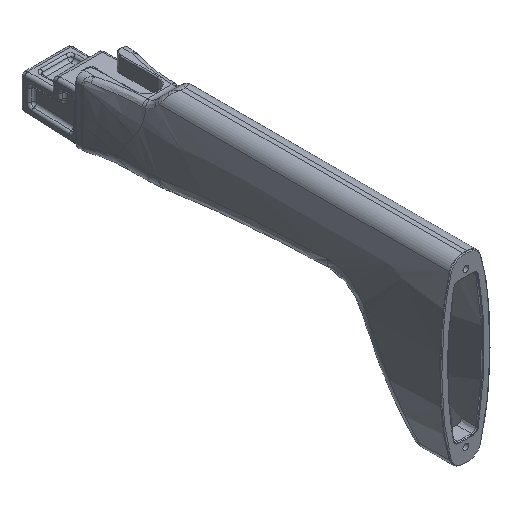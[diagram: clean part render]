
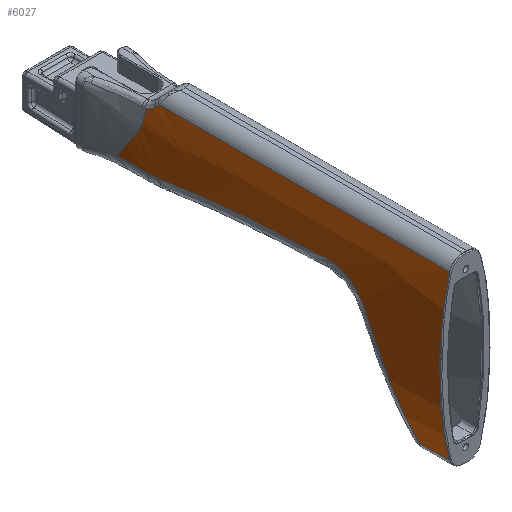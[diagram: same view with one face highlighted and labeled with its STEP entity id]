
A CAD part, isometric view. The second image highlights one B-rep face of the part: STEP entity #6027.
In plain terms, the highlighted free-form (B-spline) face has degree [1, 2] with [2, 5] control points.
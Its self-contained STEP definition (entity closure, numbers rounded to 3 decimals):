
#101=B_SPLINE_CURVE_WITH_KNOTS('',3,(#11541,#11542,#11543,#11544),
 .UNSPECIFIED.,.F.,.F.,(4,4),(-0.253,0.),.UNSPECIFIED.);
#102=B_SPLINE_CURVE_WITH_KNOTS('',3,(#11589,#11590,#11591,#11592,#11593,
#11594,#11595),.UNSPECIFIED.,.F.,.F.,(4,1,1,1,4),(-6.528,-5.596,
-4.663,-2.798,0.),.UNSPECIFIED.);
#103=B_SPLINE_CURVE_WITH_KNOTS('',3,(#11634,#11635,#11636,#11637,#11638,
#11639),.UNSPECIFIED.,.F.,.F.,(4,1,1,4),(-3.312,-2.366,
-1.419,0.),.UNSPECIFIED.);
#104=B_SPLINE_CURVE_WITH_KNOTS('',3,(#11666,#11667,#11668,#11669),
 .UNSPECIFIED.,.F.,.F.,(4,4),(-10.9,0.),.UNSPECIFIED.);
#105=B_SPLINE_CURVE_WITH_KNOTS('',3,(#11696,#11697,#11698,#11699),
 .UNSPECIFIED.,.F.,.F.,(4,4),(-0.712,0.),.UNSPECIFIED.);
#106=B_SPLINE_CURVE_WITH_KNOTS('',3,(#11724,#11725,#11726,#11727,#11728),
 .UNSPECIFIED.,.F.,.F.,(4,1,4),(23.985,24.996,26.344),
 .UNSPECIFIED.);
#107=B_SPLINE_CURVE_WITH_KNOTS('',3,(#11758,#11759,#11760,#11761,#11762,
#11763),.UNSPECIFIED.,.F.,.F.,(4,1,1,4),(0.,0.978,2.933,
3.125),.UNSPECIFIED.);
#108=B_SPLINE_CURVE_WITH_KNOTS('',3,(#11785,#11786,#11787,#11788),
 .UNSPECIFIED.,.F.,.F.,(4,4),(-0.662,-0.338),
 .UNSPECIFIED.);
#109=B_SPLINE_CURVE_WITH_KNOTS('',3,(#11789,#11790,#11791,#11792),
 .UNSPECIFIED.,.F.,.F.,(4,4),(-0.338,0.),.UNSPECIFIED.);
#124=B_SPLINE_CURVE_WITH_KNOTS('',3,(#12249,#12250,#12251,#12252,#12253,
#12254,#12255,#12256,#12257,#12258,#12259),.UNSPECIFIED.,.F.,.F.,(4,1,1,
1,1,1,1,1,4),(0.,0.763,1.525,3.05,4.575,
7.626,9.151,9.913,10.676),
 .UNSPECIFIED.);
#488=(
BOUNDED_SURFACE()
B_SPLINE_SURFACE(1,2,((#12238,#12239,#12240,#12241,#12242),(#12243,#12244,
#12245,#12246,#12247)),.UNSPECIFIED.,.F.,.F.,.F.)
B_SPLINE_SURFACE_WITH_KNOTS((2,2),(3,2,3),(0.041,3.152),
(-2.476,-1.571,-0.665),.UNSPECIFIED.)
GEOMETRIC_REPRESENTATION_ITEM()
RATIONAL_B_SPLINE_SURFACE(((1.,0.899,1.,0.899,1.),
(1.,0.899,1.,0.899,1.)))
REPRESENTATION_ITEM('')
SURFACE()
);
#880=FACE_OUTER_BOUND('',#1303,.T.);
#1303=EDGE_LOOP('',(#4921,#4922,#4923,#4924,#4925,#4926,#4927,#4928,#4929,
#4930,#4931,#4932,#4933));
#1636=LINE('',#11702,#1891);
#1640=LINE('',#12236,#1895);
#1642=LINE('',#12260,#1897);
#1891=VECTOR('',#7911,10.);
#1895=VECTOR('',#7957,10.);
#1897=VECTOR('',#7959,10.);
#2610=VERTEX_POINT('',#10348);
#2615=VERTEX_POINT('',#10564);
#2659=VERTEX_POINT('',#11513);
#2661=VERTEX_POINT('',#11538);
#2662=VERTEX_POINT('',#11540);
#2663=VERTEX_POINT('',#11588);
#2664=VERTEX_POINT('',#11633);
#2665=VERTEX_POINT('',#11665);
#2666=VERTEX_POINT('',#11695);
#2667=VERTEX_POINT('',#11723);
#2668=VERTEX_POINT('',#11784);
#2684=VERTEX_POINT('',#12233);
#2686=VERTEX_POINT('',#12248);
#3407=EDGE_CURVE('',#2661,#2662,#101,.T.);
#3409=EDGE_CURVE('',#2659,#2663,#102,.T.);
#3411=EDGE_CURVE('',#2663,#2664,#103,.T.);
#3413=EDGE_CURVE('',#2664,#2665,#104,.T.);
#3415=EDGE_CURVE('',#2665,#2666,#105,.T.);
#3417=EDGE_CURVE('',#2666,#2610,#1636,.T.);
#3418=EDGE_CURVE('',#2610,#2667,#106,.T.);
#3420=EDGE_CURVE('',#2667,#2615,#107,.T.);
#3421=EDGE_CURVE('',#2615,#2668,#108,.T.);
#3422=EDGE_CURVE('',#2668,#2661,#109,.T.);
#3455=EDGE_CURVE('',#2659,#2684,#1640,.T.);
#3457=EDGE_CURVE('',#2686,#2684,#124,.T.);
#3458=EDGE_CURVE('',#2686,#2662,#1642,.T.);
#4921=ORIENTED_EDGE('',*,*,#3421,.F.);
#4922=ORIENTED_EDGE('',*,*,#3420,.F.);
#4923=ORIENTED_EDGE('',*,*,#3418,.F.);
#4924=ORIENTED_EDGE('',*,*,#3417,.F.);
#4925=ORIENTED_EDGE('',*,*,#3415,.F.);
#4926=ORIENTED_EDGE('',*,*,#3413,.F.);
#4927=ORIENTED_EDGE('',*,*,#3411,.F.);
#4928=ORIENTED_EDGE('',*,*,#3409,.F.);
#4929=ORIENTED_EDGE('',*,*,#3455,.T.);
#4930=ORIENTED_EDGE('',*,*,#3457,.F.);
#4931=ORIENTED_EDGE('',*,*,#3458,.T.);
#4932=ORIENTED_EDGE('',*,*,#3407,.F.);
#4933=ORIENTED_EDGE('',*,*,#3422,.F.);
#6027=ADVANCED_FACE('',(#880),#488,.T.);
#7911=DIRECTION('',(0.,1.,0.));
#7957=DIRECTION('',(0.,-1.,0.));
#7959=DIRECTION('',(0.,1.,0.));
#10348=CARTESIAN_POINT('',(-15.76,-485.341,96.708));
#10564=CARTESIAN_POINT('',(-11.416,-499.135,128.202));
#11513=CARTESIAN_POINT('',(-10.031,-674.92,27.353));
#11538=CARTESIAN_POINT('',(-10.569,-504.818,131.424));
#11540=CARTESIAN_POINT('',(-10.031,-506.567,133.253));
#11541=CARTESIAN_POINT('Ctrl Pts',(-10.569,-504.818,
131.424));
#11542=CARTESIAN_POINT('Ctrl Pts',(-10.398,-505.402,132.033));
#11543=CARTESIAN_POINT('Ctrl Pts',(-10.219,-505.985,
132.643));
#11544=CARTESIAN_POINT('Ctrl Pts',(-10.031,-506.567,133.253));
#11588=CARTESIAN_POINT('',(-16.12,-647.054,88.811));
#11589=CARTESIAN_POINT('Ctrl Pts',(-10.031,-674.92,27.353));
#11590=CARTESIAN_POINT('Ctrl Pts',(-10.976,-673.632,
30.426));
#11591=CARTESIAN_POINT('Ctrl Pts',(-12.421,-671.02,
36.399));
#11592=CARTESIAN_POINT('Ctrl Pts',(-14.446,-665.738,
48.158));
#11593=CARTESIAN_POINT('Ctrl Pts',(-16.163,-657.746,
65.617));
#11594=CARTESIAN_POINT('Ctrl Pts',(-16.387,-651.061,80.106));
#11595=CARTESIAN_POINT('Ctrl Pts',(-16.12,-647.054,
88.811));
#11633=CARTESIAN_POINT('',(-15.023,-620.438,105.958));
#11634=CARTESIAN_POINT('Ctrl Pts',(-16.12,-647.054,
88.811));
#11635=CARTESIAN_POINT('Ctrl Pts',(-16.029,-645.699,
91.755));
#11636=CARTESIAN_POINT('Ctrl Pts',(-15.766,-642.052,97.18));
#11637=CARTESIAN_POINT('Ctrl Pts',(-15.225,-633.073,
104.094));
#11638=CARTESIAN_POINT('Ctrl Pts',(-15.016,-625.169,106.031));
#11639=CARTESIAN_POINT('Ctrl Pts',(-15.023,-620.438,
105.958));
#11665=CARTESIAN_POINT('',(-15.728,-511.831,97.222));
#11666=CARTESIAN_POINT('Ctrl Pts',(-15.023,-620.438,
105.958));
#11667=CARTESIAN_POINT('Ctrl Pts',(-15.079,-584.107,
105.394));
#11668=CARTESIAN_POINT('Ctrl Pts',(-15.399,-547.811,102.464));
#11669=CARTESIAN_POINT('Ctrl Pts',(-15.728,-511.831,
97.222));
#11695=CARTESIAN_POINT('',(-15.76,-504.734,96.708));
#11696=CARTESIAN_POINT('Ctrl Pts',(-15.728,-511.831,
97.222));
#11697=CARTESIAN_POINT('Ctrl Pts',(-15.75,-509.481,
96.88));
#11698=CARTESIAN_POINT('Ctrl Pts',(-15.76,-507.108,
96.708));
#11699=CARTESIAN_POINT('Ctrl Pts',(-15.76,-504.734,
96.708));
#11702=CARTESIAN_POINT('',(-15.76,-697.501,96.708));
#11723=CARTESIAN_POINT('',(-14.433,-494.201,111.229));
#11724=CARTESIAN_POINT('Ctrl Pts',(-15.76,-485.341,
96.708));
#11725=CARTESIAN_POINT('Ctrl Pts',(-15.626,-486.392,
98.922));
#11726=CARTESIAN_POINT('Ctrl Pts',(-15.251,-489.155,
103.977));
#11727=CARTESIAN_POINT('Ctrl Pts',(-14.754,-492.311,
108.661));
#11728=CARTESIAN_POINT('Ctrl Pts',(-14.433,-494.201,
111.229));
#11758=CARTESIAN_POINT('Ctrl Pts',(-14.433,-494.201,
111.229));
#11759=CARTESIAN_POINT('Ctrl Pts',(-14.201,-495.568,
113.087));
#11760=CARTESIAN_POINT('Ctrl Pts',(-13.407,-498.802,
118.817));
#11761=CARTESIAN_POINT('Ctrl Pts',(-12.296,-499.637,124.546));
#11762=CARTESIAN_POINT('Ctrl Pts',(-11.489,-499.184,
127.907));
#11763=CARTESIAN_POINT('Ctrl Pts',(-11.417,-499.136,
128.202));
#11784=CARTESIAN_POINT('',(-11.125,-502.153,129.36));
#11785=CARTESIAN_POINT('Ctrl Pts',(-11.416,-499.135,128.202));
#11786=CARTESIAN_POINT('Ctrl Pts',(-11.357,-500.19,128.439));
#11787=CARTESIAN_POINT('Ctrl Pts',(-11.261,-501.207,
128.835));
#11788=CARTESIAN_POINT('Ctrl Pts',(-11.125,-502.151,
129.364));
#11789=CARTESIAN_POINT('Ctrl Pts',(-11.125,-502.151,
129.364));
#11790=CARTESIAN_POINT('Ctrl Pts',(-10.984,-503.134,
129.915));
#11791=CARTESIAN_POINT('Ctrl Pts',(-10.799,-504.037,
130.611));
#11792=CARTESIAN_POINT('Ctrl Pts',(-10.569,-504.818,
131.424));
#12233=CARTESIAN_POINT('',(-10.031,-694.735,27.353));
#12236=CARTESIAN_POINT('',(-10.031,-697.501,27.353));
#12238=CARTESIAN_POINT('Ctrl Pts',(-10.031,-694.735,133.253));
#12239=CARTESIAN_POINT('Ctrl Pts',(-16.25,-694.735,
113.043));
#12240=CARTESIAN_POINT('Ctrl Pts',(-16.25,-694.735,
80.303));
#12241=CARTESIAN_POINT('Ctrl Pts',(-16.25,-694.735,
47.563));
#12242=CARTESIAN_POINT('Ctrl Pts',(-10.031,-694.735,27.353));
#12243=CARTESIAN_POINT('Ctrl Pts',(-10.031,-485.341,133.253));
#12244=CARTESIAN_POINT('Ctrl Pts',(-16.25,-485.341,
113.043));
#12245=CARTESIAN_POINT('Ctrl Pts',(-16.25,-485.341,
80.303));
#12246=CARTESIAN_POINT('Ctrl Pts',(-16.25,-485.341,
47.563));
#12247=CARTESIAN_POINT('Ctrl Pts',(-10.031,-485.341,27.353));
#12248=CARTESIAN_POINT('',(-10.031,-694.735,133.253));
#12249=CARTESIAN_POINT('Ctrl Pts',(-10.031,-694.735,133.253));
#12250=CARTESIAN_POINT('Ctrl Pts',(-10.782,-694.735,
130.811));
#12251=CARTESIAN_POINT('Ctrl Pts',(-12.045,-694.735,
125.859));
#12252=CARTESIAN_POINT('Ctrl Pts',(-13.936,-694.735,
115.844));
#12253=CARTESIAN_POINT('Ctrl Pts',(-15.446,-694.735,
103.181));
#12254=CARTESIAN_POINT('Ctrl Pts',(-16.558,-694.735,82.854));
#12255=CARTESIAN_POINT('Ctrl Pts',(-16.032,-694.735,
62.458));
#12256=CARTESIAN_POINT('Ctrl Pts',(-13.94,-694.735,
44.771));
#12257=CARTESIAN_POINT('Ctrl Pts',(-12.043,-694.735,
34.745));
#12258=CARTESIAN_POINT('Ctrl Pts',(-10.782,-694.735,
29.795));
#12259=CARTESIAN_POINT('Ctrl Pts',(-10.031,-694.735,27.353));
#12260=CARTESIAN_POINT('',(-10.031,-697.501,133.253));
